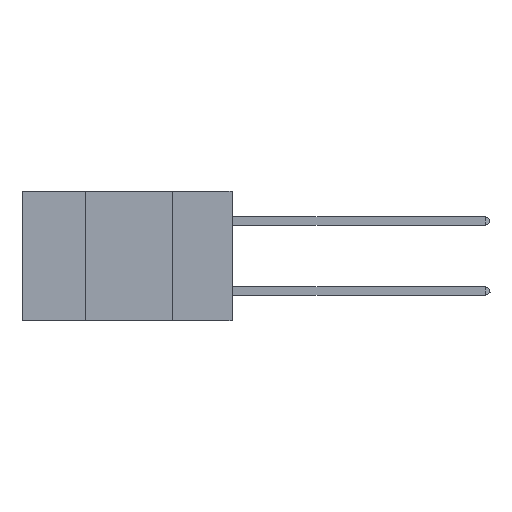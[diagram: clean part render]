
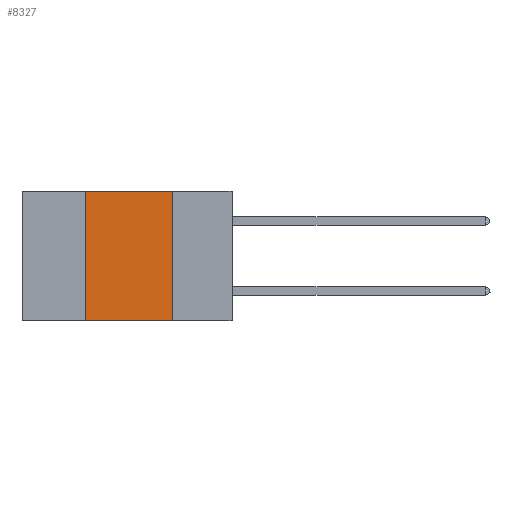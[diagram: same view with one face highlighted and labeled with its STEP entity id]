
A CAD part, left-side view. The second image highlights one B-rep face of the part: STEP entity #8327.
In plain terms, the highlighted planar face has unit normal (-1, 0, 0).
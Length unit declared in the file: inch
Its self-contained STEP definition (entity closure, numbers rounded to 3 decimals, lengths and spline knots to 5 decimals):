
#568 = VERTEX_POINT ( 'NONE', #14370 ) ;
#1512 = LINE ( 'NONE', #19144, #15947 ) ;
#2855 = CARTESIAN_POINT ( 'NONE',  ( 0., 0.42, -0.37 ) ) ;
#3165 = ORIENTED_EDGE ( 'NONE', *, *, #13194, .F. ) ;
#3820 = CARTESIAN_POINT ( 'NONE',  ( 0., 0.17, 0. ) ) ;
#4604 = EDGE_LOOP ( 'NONE', ( #19564, #9589, #3165, #18519 ) ) ;
#4655 = FACE_OUTER_BOUND ( 'NONE', #4604, .T. ) ;
#6422 = CARTESIAN_POINT ( 'NONE',  ( 0., 0.6, 0. ) ) ;
#6681 = EDGE_CURVE ( 'NONE', #17323, #19687, #1512, .T. ) ;
#7096 = CARTESIAN_POINT ( 'NONE',  ( 0., 0.6, 0. ) ) ;
#7616 = VECTOR ( 'NONE', #11017, 39.37008 ) ;
#7845 = CARTESIAN_POINT ( 'NONE',  ( 0., 0.42, 0. ) ) ;
#8185 = VECTOR ( 'NONE', #19221, 39.37008 ) ;
#8322 = PLANE ( 'NONE',  #13696 ) ;
#8327 = ADVANCED_FACE ( 'NONE', ( #4655 ), #8322, .F. ) ;
#8704 = VERTEX_POINT ( 'NONE', #16257 ) ;
#9589 = ORIENTED_EDGE ( 'NONE', *, *, #12289, .F. ) ;
#10282 = DIRECTION ( 'NONE',  ( 0., -1., 0. ) ) ;
#11017 = DIRECTION ( 'NONE',  ( 0., 0., 1. ) ) ;
#11639 = DIRECTION ( 'NONE',  ( 1., 0., 0. ) ) ;
#12012 = CARTESIAN_POINT ( 'NONE',  ( 0., 0.17, -0.37 ) ) ;
#12289 = EDGE_CURVE ( 'NONE', #568, #8704, #18997, .T. ) ;
#12299 = LINE ( 'NONE', #3820, #8185 ) ;
#13194 = EDGE_CURVE ( 'NONE', #17323, #568, #15528, .T. ) ;
#13696 = AXIS2_PLACEMENT_3D ( 'NONE', #7096, #11639, #19282 ) ;
#14370 = CARTESIAN_POINT ( 'NONE',  ( 0., 0.42, 0. ) ) ;
#15528 = LINE ( 'NONE', #7845, #7616 ) ;
#15947 = VECTOR ( 'NONE', #10282, 39.37008 ) ;
#16257 = CARTESIAN_POINT ( 'NONE',  ( 0., 0.17, 0. ) ) ;
#17323 = VERTEX_POINT ( 'NONE', #2855 ) ;
#18119 = EDGE_CURVE ( 'NONE', #8704, #19687, #12299, .T. ) ;
#18519 = ORIENTED_EDGE ( 'NONE', *, *, #6681, .T. ) ;
#18764 = VECTOR ( 'NONE', #18899, 39.37008 ) ;
#18899 = DIRECTION ( 'NONE',  ( 0., -1., 0. ) ) ;
#18997 = LINE ( 'NONE', #6422, #18764 ) ;
#19144 = CARTESIAN_POINT ( 'NONE',  ( 0., 0.6, -0.37 ) ) ;
#19221 = DIRECTION ( 'NONE',  ( 0., 0., -1. ) ) ;
#19282 = DIRECTION ( 'NONE',  ( 0., 0., -1. ) ) ;
#19564 = ORIENTED_EDGE ( 'NONE', *, *, #18119, .F. ) ;
#19687 = VERTEX_POINT ( 'NONE', #12012 ) ;
